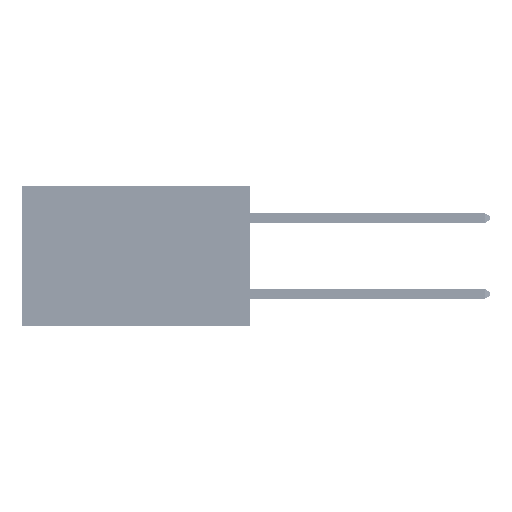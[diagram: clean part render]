
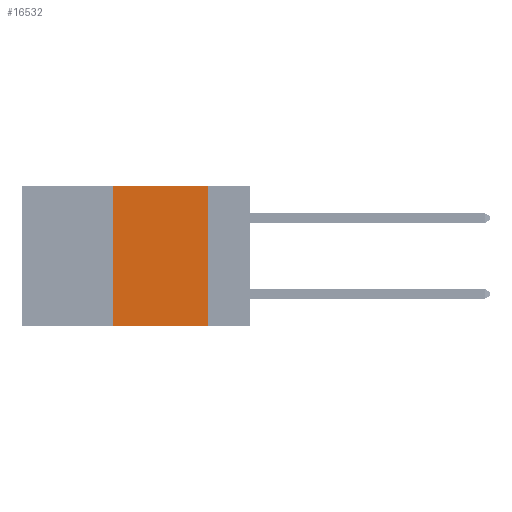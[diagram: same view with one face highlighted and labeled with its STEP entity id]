
A CAD part, left-side view. The second image highlights one B-rep face of the part: STEP entity #16532.
In plain terms, the highlighted planar face has unit normal (-1, 0, 0).
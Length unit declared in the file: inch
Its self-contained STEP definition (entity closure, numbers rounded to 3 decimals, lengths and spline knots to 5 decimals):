
#748 = ORIENTED_EDGE ( 'NONE', *, *, #30100, .F. ) ;
#931 = VERTEX_POINT ( 'NONE', #18929 ) ;
#2391 = PLANE ( 'NONE',  #18308 ) ;
#3513 = DIRECTION ( 'NONE',  ( 0., -1., 0. ) ) ;
#3944 = VERTEX_POINT ( 'NONE', #9787 ) ;
#4309 = CARTESIAN_POINT ( 'NONE',  ( 0., 0.11, 0. ) ) ;
#4988 = DIRECTION ( 'NONE',  ( 0., -1., 0. ) ) ;
#7620 = CARTESIAN_POINT ( 'NONE',  ( 0., 0.6, 0. ) ) ;
#9787 = CARTESIAN_POINT ( 'NONE',  ( 0., 0.11, -0.37 ) ) ;
#9898 = DIRECTION ( 'NONE',  ( 0., 0., -1. ) ) ;
#10459 = EDGE_CURVE ( 'NONE', #931, #11865, #25685, .T. ) ;
#11600 = VECTOR ( 'NONE', #18824, 39.37008 ) ;
#11865 = VERTEX_POINT ( 'NONE', #33244 ) ;
#14218 = EDGE_LOOP ( 'NONE', ( #36102, #748, #25003, #43058 ) ) ;
#15470 = CARTESIAN_POINT ( 'NONE',  ( 0., 0.36, 0. ) ) ;
#16532 = ADVANCED_FACE ( 'NONE', ( #39191 ), #2391, .F. ) ;
#17161 = CARTESIAN_POINT ( 'NONE',  ( 0., 0.6, 0. ) ) ;
#18308 = AXIS2_PLACEMENT_3D ( 'NONE', #17161, #43069, #9898 ) ;
#18824 = DIRECTION ( 'NONE',  ( 0., 0., -1. ) ) ;
#18929 = CARTESIAN_POINT ( 'NONE',  ( 0., 0.36, -0.37 ) ) ;
#20179 = EDGE_CURVE ( 'NONE', #23306, #3944, #22454, .T. ) ;
#22132 = LINE ( 'NONE', #7620, #38422 ) ;
#22270 = DIRECTION ( 'NONE',  ( 0., 0., 1. ) ) ;
#22454 = LINE ( 'NONE', #4309, #11600 ) ;
#23306 = VERTEX_POINT ( 'NONE', #41959 ) ;
#25003 = ORIENTED_EDGE ( 'NONE', *, *, #10459, .F. ) ;
#25685 = LINE ( 'NONE', #15470, #46652 ) ;
#30100 = EDGE_CURVE ( 'NONE', #11865, #23306, #22132, .T. ) ;
#33244 = CARTESIAN_POINT ( 'NONE',  ( 0., 0.36, 0. ) ) ;
#36102 = ORIENTED_EDGE ( 'NONE', *, *, #20179, .F. ) ;
#38143 = CARTESIAN_POINT ( 'NONE',  ( 0., 0.6, -0.37 ) ) ;
#38422 = VECTOR ( 'NONE', #3513, 39.37008 ) ;
#39191 = FACE_OUTER_BOUND ( 'NONE', #14218, .T. ) ;
#41082 = LINE ( 'NONE', #38143, #44850 ) ;
#41959 = CARTESIAN_POINT ( 'NONE',  ( 0., 0.11, 0. ) ) ;
#43036 = EDGE_CURVE ( 'NONE', #931, #3944, #41082, .T. ) ;
#43058 = ORIENTED_EDGE ( 'NONE', *, *, #43036, .T. ) ;
#43069 = DIRECTION ( 'NONE',  ( 1., 0., 0. ) ) ;
#44850 = VECTOR ( 'NONE', #4988, 39.37008 ) ;
#46652 = VECTOR ( 'NONE', #22270, 39.37008 ) ;
